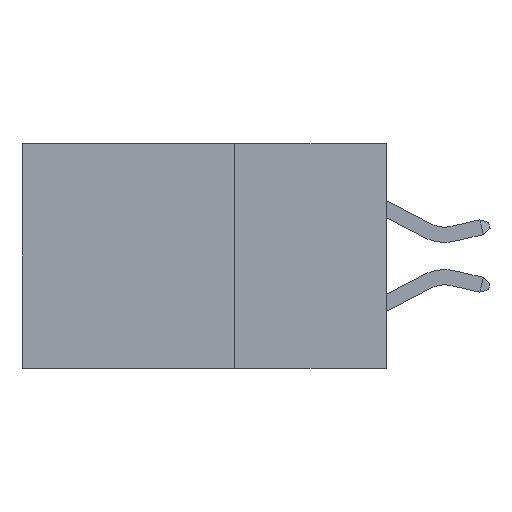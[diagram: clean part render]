
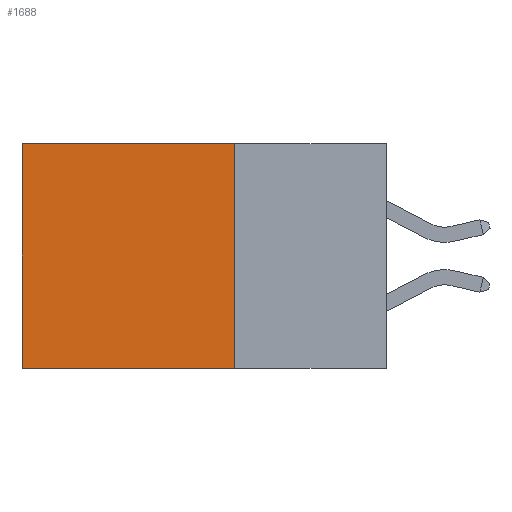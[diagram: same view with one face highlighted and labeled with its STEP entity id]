
A CAD part, left-side view. The second image highlights one B-rep face of the part: STEP entity #1688.
In plain terms, the highlighted planar face has unit normal (-1, 0, 0).
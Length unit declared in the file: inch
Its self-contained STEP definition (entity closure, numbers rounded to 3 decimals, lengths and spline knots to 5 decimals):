
#1688 = ADVANCED_FACE ( 'NONE', ( #2247 ), #18271, .F. ) ;
#2247 = FACE_OUTER_BOUND ( 'NONE', #23455, .T. ) ;
#2361 = CARTESIAN_POINT ( 'NONE',  ( 0.298, 0.6, -0.37 ) ) ;
#3850 = EDGE_CURVE ( 'NONE', #4835, #17296, #15884, .T. ) ;
#4174 = CARTESIAN_POINT ( 'NONE',  ( 0.298, 0.25, 0. ) ) ;
#4835 = VERTEX_POINT ( 'NONE', #14741 ) ;
#5354 = DIRECTION ( 'NONE',  ( 0., 1., 0. ) ) ;
#5970 = CARTESIAN_POINT ( 'NONE',  ( 0.298, 0.25, 0. ) ) ;
#7451 = CARTESIAN_POINT ( 'NONE',  ( 0.298, 0.6, 0. ) ) ;
#7859 = VECTOR ( 'NONE', #21159, 39.37008 ) ;
#8407 = EDGE_CURVE ( 'NONE', #20017, #12827, #19369, .T. ) ;
#8707 = ORIENTED_EDGE ( 'NONE', *, *, #3850, .F. ) ;
#10033 = LINE ( 'NONE', #7451, #15150 ) ;
#10818 = DIRECTION ( 'NONE',  ( 0., 1., 0. ) ) ;
#11866 = ORIENTED_EDGE ( 'NONE', *, *, #8407, .T. ) ;
#12827 = VERTEX_POINT ( 'NONE', #21695 ) ;
#12852 = ORIENTED_EDGE ( 'NONE', *, *, #18054, .T. ) ;
#13614 = VECTOR ( 'NONE', #10818, 39.37008 ) ;
#14032 = DIRECTION ( 'NONE',  ( 0., 0., -1. ) ) ;
#14741 = CARTESIAN_POINT ( 'NONE',  ( 0.298, 0.25, -0.37 ) ) ;
#15150 = VECTOR ( 'NONE', #14032, 39.37008 ) ;
#15884 = LINE ( 'NONE', #21524, #26697 ) ;
#17296 = VERTEX_POINT ( 'NONE', #2361 ) ;
#18054 = EDGE_CURVE ( 'NONE', #12827, #17296, #10033, .T. ) ;
#18095 = LINE ( 'NONE', #5970, #7859 ) ;
#18098 = DIRECTION ( 'NONE',  ( 0., 0., -1. ) ) ;
#18193 = CARTESIAN_POINT ( 'NONE',  ( 0.298, 0.25, 0. ) ) ;
#18271 = PLANE ( 'NONE',  #27444 ) ;
#19369 = LINE ( 'NONE', #4174, #13614 ) ;
#20017 = VERTEX_POINT ( 'NONE', #26783 ) ;
#21159 = DIRECTION ( 'NONE',  ( 0., 0., -1. ) ) ;
#21524 = CARTESIAN_POINT ( 'NONE',  ( 0.298, 0.25, -0.37 ) ) ;
#21695 = CARTESIAN_POINT ( 'NONE',  ( 0.298, 0.6, 0. ) ) ;
#22220 = DIRECTION ( 'NONE',  ( 1., 0., 0. ) ) ;
#23444 = EDGE_CURVE ( 'NONE', #20017, #4835, #18095, .T. ) ;
#23455 = EDGE_LOOP ( 'NONE', ( #12852, #8707, #25957, #11866 ) ) ;
#25957 = ORIENTED_EDGE ( 'NONE', *, *, #23444, .F. ) ;
#26697 = VECTOR ( 'NONE', #5354, 39.37008 ) ;
#26783 = CARTESIAN_POINT ( 'NONE',  ( 0.298, 0.25, 0. ) ) ;
#27444 = AXIS2_PLACEMENT_3D ( 'NONE', #18193, #22220, #18098 ) ;
